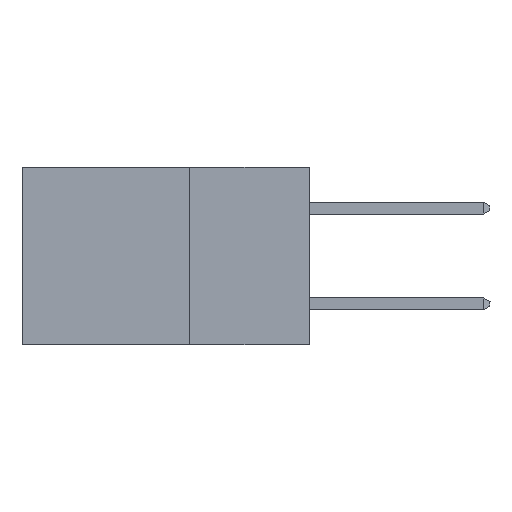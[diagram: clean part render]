
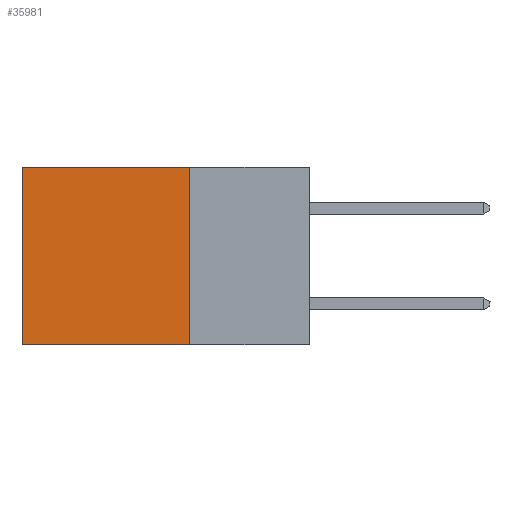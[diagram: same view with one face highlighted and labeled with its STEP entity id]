
A CAD part, left-side view. The second image highlights one B-rep face of the part: STEP entity #35981.
In plain terms, the highlighted planar face has unit normal (-1, 0, 0).
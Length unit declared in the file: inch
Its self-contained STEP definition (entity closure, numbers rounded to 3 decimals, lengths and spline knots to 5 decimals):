
#485 = VECTOR ( 'NONE', #37806, 39.37008 ) ;
#528 = CARTESIAN_POINT ( 'NONE',  ( 0.2875, 0.25, -0.37 ) ) ;
#1117 = LINE ( 'NONE', #14244, #9588 ) ;
#2349 = EDGE_CURVE ( 'NONE', #38523, #40680, #37114, .T. ) ;
#4416 = ORIENTED_EDGE ( 'NONE', *, *, #34444, .F. ) ;
#6259 = DIRECTION ( 'NONE',  ( 1., 0., 0. ) ) ;
#7835 = CARTESIAN_POINT ( 'NONE',  ( 0.2875, 0.25, -0.37 ) ) ;
#9588 = VECTOR ( 'NONE', #27609, 39.37008 ) ;
#10323 = PLANE ( 'NONE',  #26205 ) ;
#11766 = VECTOR ( 'NONE', #23976, 39.37008 ) ;
#13806 = ORIENTED_EDGE ( 'NONE', *, *, #37819, .T. ) ;
#14244 = CARTESIAN_POINT ( 'NONE',  ( 0.2875, 0.25, 0. ) ) ;
#14884 = CARTESIAN_POINT ( 'NONE',  ( 0.2875, 0.6, 0. ) ) ;
#19399 = DIRECTION ( 'NONE',  ( 0., 0., -1. ) ) ;
#19566 = DIRECTION ( 'NONE',  ( 0., 0., -1. ) ) ;
#20717 = VERTEX_POINT ( 'NONE', #26627 ) ;
#22220 = CARTESIAN_POINT ( 'NONE',  ( 0.2875, 0.6, -0.37 ) ) ;
#23225 = CARTESIAN_POINT ( 'NONE',  ( 0.2875, 0.6, 0. ) ) ;
#23482 = CARTESIAN_POINT ( 'NONE',  ( 0.2875, 0.25, 0. ) ) ;
#23976 = DIRECTION ( 'NONE',  ( 0., 1., 0. ) ) ;
#26205 = AXIS2_PLACEMENT_3D ( 'NONE', #23482, #6259, #19399 ) ;
#26627 = CARTESIAN_POINT ( 'NONE',  ( 0.2875, 0.25, 0. ) ) ;
#27609 = DIRECTION ( 'NONE',  ( 0., 0., -1. ) ) ;
#27900 = ORIENTED_EDGE ( 'NONE', *, *, #2349, .F. ) ;
#29095 = EDGE_CURVE ( 'NONE', #20717, #39150, #41239, .T. ) ;
#34444 = EDGE_CURVE ( 'NONE', #20717, #38523, #1117, .T. ) ;
#35981 = ADVANCED_FACE ( 'NONE', ( #39618 ), #10323, .F. ) ;
#36149 = LINE ( 'NONE', #23225, #41454 ) ;
#37114 = LINE ( 'NONE', #7835, #11766 ) ;
#37806 = DIRECTION ( 'NONE',  ( 0., 1., 0. ) ) ;
#37819 = EDGE_CURVE ( 'NONE', #39150, #40680, #36149, .T. ) ;
#38523 = VERTEX_POINT ( 'NONE', #528 ) ;
#39150 = VERTEX_POINT ( 'NONE', #14884 ) ;
#39261 = ORIENTED_EDGE ( 'NONE', *, *, #29095, .T. ) ;
#39618 = FACE_OUTER_BOUND ( 'NONE', #40964, .T. ) ;
#40680 = VERTEX_POINT ( 'NONE', #22220 ) ;
#40825 = CARTESIAN_POINT ( 'NONE',  ( 0.2875, 0.25, 0. ) ) ;
#40964 = EDGE_LOOP ( 'NONE', ( #13806, #27900, #4416, #39261 ) ) ;
#41239 = LINE ( 'NONE', #40825, #485 ) ;
#41454 = VECTOR ( 'NONE', #19566, 39.37008 ) ;
